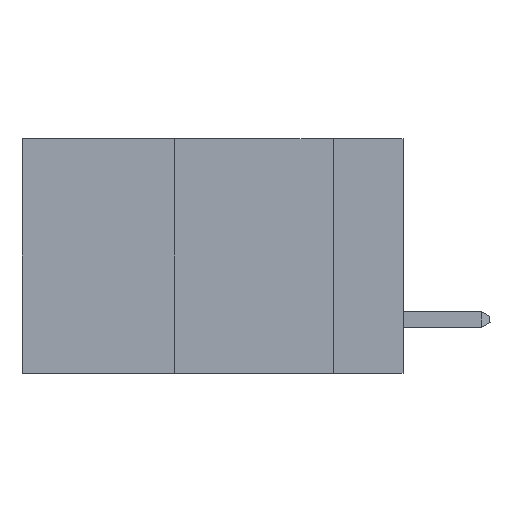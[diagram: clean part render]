
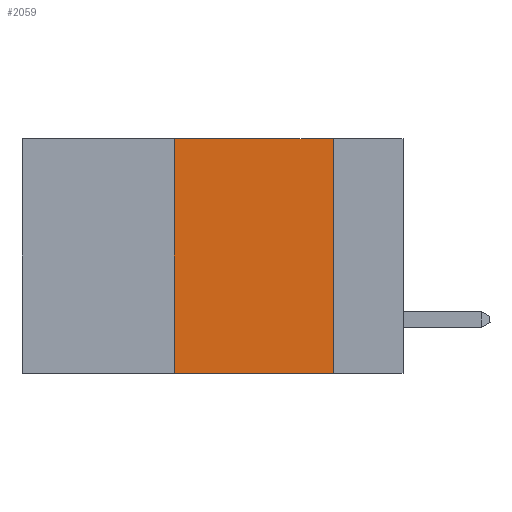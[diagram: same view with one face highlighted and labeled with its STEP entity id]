
A CAD part, left-side view. The second image highlights one B-rep face of the part: STEP entity #2059.
In plain terms, the highlighted planar face has unit normal (-1, 0, 0).
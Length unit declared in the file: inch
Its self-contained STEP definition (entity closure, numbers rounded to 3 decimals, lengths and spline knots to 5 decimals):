
#775 = EDGE_CURVE ( 'NONE', #2971, #2324, #7943, .T. ) ;
#1006 = EDGE_CURVE ( 'NONE', #2324, #10578, #2746, .T. ) ;
#1078 = CARTESIAN_POINT ( 'NONE',  ( 0., 0.36, -0.37 ) ) ;
#1158 = EDGE_LOOP ( 'NONE', ( #5345, #2093, #1997, #7191 ) ) ;
#1317 = FACE_OUTER_BOUND ( 'NONE', #1158, .T. ) ;
#1342 = VECTOR ( 'NONE', #8039, 39.37008 ) ;
#1638 = DIRECTION ( 'NONE',  ( 1., 0., 0. ) ) ;
#1997 = ORIENTED_EDGE ( 'NONE', *, *, #6664, .F. ) ;
#2059 = ADVANCED_FACE ( 'NONE', ( #1317 ), #6873, .F. ) ;
#2093 = ORIENTED_EDGE ( 'NONE', *, *, #775, .F. ) ;
#2097 = CARTESIAN_POINT ( 'NONE',  ( 0., 0.36, 0. ) ) ;
#2324 = VERTEX_POINT ( 'NONE', #8434 ) ;
#2746 = LINE ( 'NONE', #6046, #4770 ) ;
#2971 = VERTEX_POINT ( 'NONE', #8597 ) ;
#3456 = DIRECTION ( 'NONE',  ( 0., 0., -1. ) ) ;
#3547 = CARTESIAN_POINT ( 'NONE',  ( 0., 0.6, 0. ) ) ;
#4770 = VECTOR ( 'NONE', #5131, 39.37008 ) ;
#5131 = DIRECTION ( 'NONE',  ( 0., 0., -1. ) ) ;
#5345 = ORIENTED_EDGE ( 'NONE', *, *, #1006, .F. ) ;
#5488 = CARTESIAN_POINT ( 'NONE',  ( 0., 0.6, -0.37 ) ) ;
#5990 = VECTOR ( 'NONE', #10141, 39.37008 ) ;
#6046 = CARTESIAN_POINT ( 'NONE',  ( 0., 0.11, 0. ) ) ;
#6153 = VECTOR ( 'NONE', #8253, 39.37008 ) ;
#6196 = AXIS2_PLACEMENT_3D ( 'NONE', #11330, #1638, #3456 ) ;
#6664 = EDGE_CURVE ( 'NONE', #8573, #2971, #8515, .T. ) ;
#6873 = PLANE ( 'NONE',  #6196 ) ;
#7191 = ORIENTED_EDGE ( 'NONE', *, *, #7974, .T. ) ;
#7943 = LINE ( 'NONE', #3547, #5990 ) ;
#7974 = EDGE_CURVE ( 'NONE', #8573, #10578, #9445, .T. ) ;
#8039 = DIRECTION ( 'NONE',  ( 0., -1., 0. ) ) ;
#8253 = DIRECTION ( 'NONE',  ( 0., 0., 1. ) ) ;
#8434 = CARTESIAN_POINT ( 'NONE',  ( 0., 0.11, 0. ) ) ;
#8515 = LINE ( 'NONE', #2097, #6153 ) ;
#8573 = VERTEX_POINT ( 'NONE', #1078 ) ;
#8597 = CARTESIAN_POINT ( 'NONE',  ( 0., 0.36, 0. ) ) ;
#9445 = LINE ( 'NONE', #5488, #1342 ) ;
#10120 = CARTESIAN_POINT ( 'NONE',  ( 0., 0.11, -0.37 ) ) ;
#10141 = DIRECTION ( 'NONE',  ( 0., -1., 0. ) ) ;
#10578 = VERTEX_POINT ( 'NONE', #10120 ) ;
#11330 = CARTESIAN_POINT ( 'NONE',  ( 0., 0.6, 0. ) ) ;
